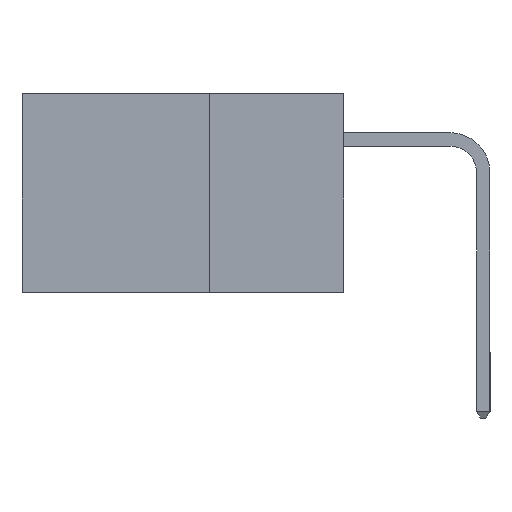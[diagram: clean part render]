
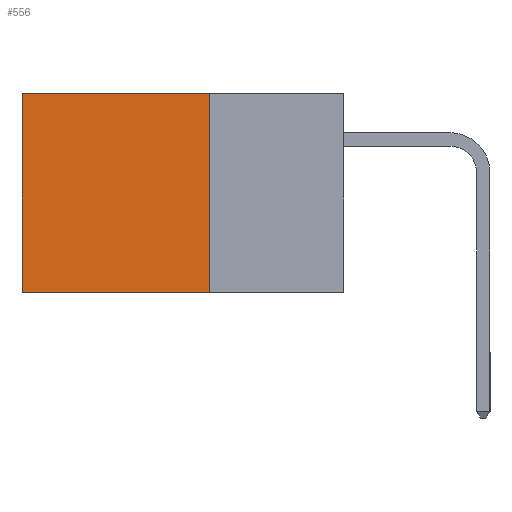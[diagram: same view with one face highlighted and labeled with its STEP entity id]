
A CAD part, left-side view. The second image highlights one B-rep face of the part: STEP entity #556.
In plain terms, the highlighted planar face has unit normal (-1, 0, 0).
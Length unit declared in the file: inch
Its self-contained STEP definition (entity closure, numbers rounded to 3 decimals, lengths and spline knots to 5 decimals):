
#164 = AXIS2_PLACEMENT_3D ( 'NONE', #10327, #1584, #2456 ) ;
#202 = FACE_OUTER_BOUND ( 'NONE', #2234, .T. ) ;
#222 = VERTEX_POINT ( 'NONE', #5488 ) ;
#556 = ADVANCED_FACE ( 'NONE', ( #202 ), #10153, .F. ) ;
#1322 = VERTEX_POINT ( 'NONE', #4390 ) ;
#1584 = DIRECTION ( 'NONE',  ( 1., 0., 0. ) ) ;
#2234 = EDGE_LOOP ( 'NONE', ( #3992, #9149, #7920, #9226 ) ) ;
#2456 = DIRECTION ( 'NONE',  ( 0., 0., -1. ) ) ;
#2782 = LINE ( 'NONE', #6483, #7797 ) ;
#2938 = VERTEX_POINT ( 'NONE', #6476 ) ;
#2952 = CARTESIAN_POINT ( 'NONE',  ( 0.298, 0.6, 0. ) ) ;
#3992 = ORIENTED_EDGE ( 'NONE', *, *, #7821, .T. ) ;
#4390 = CARTESIAN_POINT ( 'NONE',  ( 0.298, 0.6, 0. ) ) ;
#4491 = CARTESIAN_POINT ( 'NONE',  ( 0.298, 0.25, 0. ) ) ;
#4563 = VECTOR ( 'NONE', #5562, 39.37008 ) ;
#4566 = CARTESIAN_POINT ( 'NONE',  ( 0.298, 0.25, 0. ) ) ;
#5420 = DIRECTION ( 'NONE',  ( 0., 0., -1. ) ) ;
#5426 = VECTOR ( 'NONE', #5420, 39.37008 ) ;
#5488 = CARTESIAN_POINT ( 'NONE',  ( 0.298, 0.25, -0.37 ) ) ;
#5562 = DIRECTION ( 'NONE',  ( 0., 0., -1. ) ) ;
#5566 = DIRECTION ( 'NONE',  ( 0., 1., 0. ) ) ;
#5959 = LINE ( 'NONE', #4491, #6340 ) ;
#6340 = VECTOR ( 'NONE', #7734, 39.37008 ) ;
#6469 = EDGE_CURVE ( 'NONE', #222, #2938, #2782, .T. ) ;
#6476 = CARTESIAN_POINT ( 'NONE',  ( 0.298, 0.6, -0.37 ) ) ;
#6483 = CARTESIAN_POINT ( 'NONE',  ( 0.298, 0.25, -0.37 ) ) ;
#6917 = EDGE_CURVE ( 'NONE', #10354, #222, #8349, .T. ) ;
#6960 = EDGE_CURVE ( 'NONE', #10354, #1322, #5959, .T. ) ;
#7734 = DIRECTION ( 'NONE',  ( 0., 1., 0. ) ) ;
#7797 = VECTOR ( 'NONE', #5566, 39.37008 ) ;
#7821 = EDGE_CURVE ( 'NONE', #1322, #2938, #8215, .T. ) ;
#7920 = ORIENTED_EDGE ( 'NONE', *, *, #6917, .F. ) ;
#8215 = LINE ( 'NONE', #2952, #5426 ) ;
#8349 = LINE ( 'NONE', #8620, #4563 ) ;
#8620 = CARTESIAN_POINT ( 'NONE',  ( 0.298, 0.25, 0. ) ) ;
#9149 = ORIENTED_EDGE ( 'NONE', *, *, #6469, .F. ) ;
#9226 = ORIENTED_EDGE ( 'NONE', *, *, #6960, .T. ) ;
#10153 = PLANE ( 'NONE',  #164 ) ;
#10327 = CARTESIAN_POINT ( 'NONE',  ( 0.298, 0.25, 0. ) ) ;
#10354 = VERTEX_POINT ( 'NONE', #4566 ) ;
